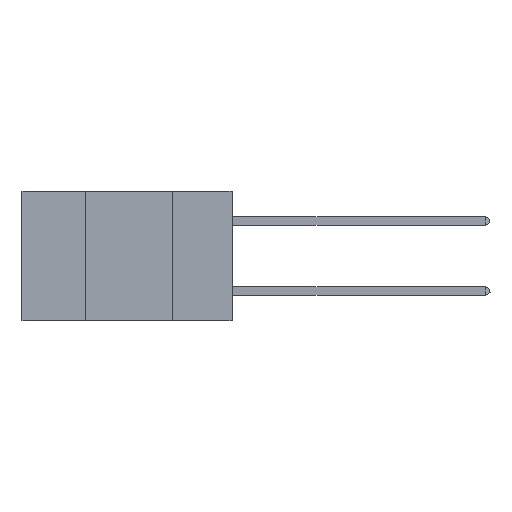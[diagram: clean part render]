
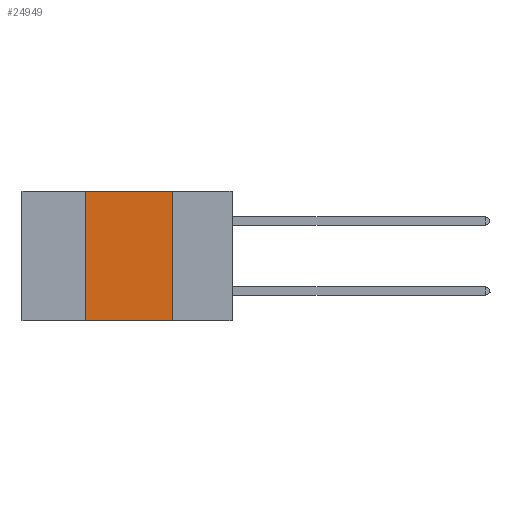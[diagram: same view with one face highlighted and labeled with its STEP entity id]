
A CAD part, left-side view. The second image highlights one B-rep face of the part: STEP entity #24949.
In plain terms, the highlighted planar face has unit normal (-1, 0, 0).
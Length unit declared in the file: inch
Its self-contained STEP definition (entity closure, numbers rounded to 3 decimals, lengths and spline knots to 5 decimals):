
#1247 = ORIENTED_EDGE ( 'NONE', *, *, #37031, .F. ) ;
#2104 = DIRECTION ( 'NONE',  ( 0., -1., 0. ) ) ;
#2487 = LINE ( 'NONE', #45721, #45930 ) ;
#5818 = CARTESIAN_POINT ( 'NONE',  ( 0., 0.6, 0. ) ) ;
#5965 = DIRECTION ( 'NONE',  ( 1., 0., 0. ) ) ;
#6819 = CARTESIAN_POINT ( 'NONE',  ( 0., 0.17, 0. ) ) ;
#7009 = ORIENTED_EDGE ( 'NONE', *, *, #16917, .T. ) ;
#8090 = CARTESIAN_POINT ( 'NONE',  ( 0., 0.17, 0. ) ) ;
#9541 = EDGE_CURVE ( 'NONE', #20435, #16058, #31429, .T. ) ;
#9655 = CARTESIAN_POINT ( 'NONE',  ( 0., 0.17, -0.37 ) ) ;
#9886 = ORIENTED_EDGE ( 'NONE', *, *, #9541, .F. ) ;
#12875 = DIRECTION ( 'NONE',  ( 0., 0., 1. ) ) ;
#13687 = CARTESIAN_POINT ( 'NONE',  ( 0., 0.42, -0.37 ) ) ;
#13893 = FACE_OUTER_BOUND ( 'NONE', #33043, .T. ) ;
#14731 = VERTEX_POINT ( 'NONE', #9655 ) ;
#15831 = VECTOR ( 'NONE', #2104, 39.37008 ) ;
#16058 = VERTEX_POINT ( 'NONE', #6819 ) ;
#16310 = EDGE_CURVE ( 'NONE', #16058, #14731, #19232, .T. ) ;
#16917 = EDGE_CURVE ( 'NONE', #30907, #14731, #37440, .T. ) ;
#19232 = LINE ( 'NONE', #8090, #39708 ) ;
#20435 = VERTEX_POINT ( 'NONE', #22971 ) ;
#22971 = CARTESIAN_POINT ( 'NONE',  ( 0., 0.42, 0. ) ) ;
#24518 = CARTESIAN_POINT ( 'NONE',  ( 0., 0.6, 0. ) ) ;
#24725 = AXIS2_PLACEMENT_3D ( 'NONE', #5818, #5965, #35308 ) ;
#24949 = ADVANCED_FACE ( 'NONE', ( #13893 ), #42811, .F. ) ;
#29490 = DIRECTION ( 'NONE',  ( 0., 0., -1. ) ) ;
#30907 = VERTEX_POINT ( 'NONE', #13687 ) ;
#31429 = LINE ( 'NONE', #24518, #37126 ) ;
#31576 = ORIENTED_EDGE ( 'NONE', *, *, #16310, .F. ) ;
#33043 = EDGE_LOOP ( 'NONE', ( #31576, #9886, #1247, #7009 ) ) ;
#35308 = DIRECTION ( 'NONE',  ( 0., 0., -1. ) ) ;
#37031 = EDGE_CURVE ( 'NONE', #30907, #20435, #2487, .T. ) ;
#37126 = VECTOR ( 'NONE', #42857, 39.37008 ) ;
#37440 = LINE ( 'NONE', #43284, #15831 ) ;
#39708 = VECTOR ( 'NONE', #29490, 39.37008 ) ;
#42811 = PLANE ( 'NONE',  #24725 ) ;
#42857 = DIRECTION ( 'NONE',  ( 0., -1., 0. ) ) ;
#43284 = CARTESIAN_POINT ( 'NONE',  ( 0., 0.6, -0.37 ) ) ;
#45721 = CARTESIAN_POINT ( 'NONE',  ( 0., 0.42, 0. ) ) ;
#45930 = VECTOR ( 'NONE', #12875, 39.37008 ) ;
